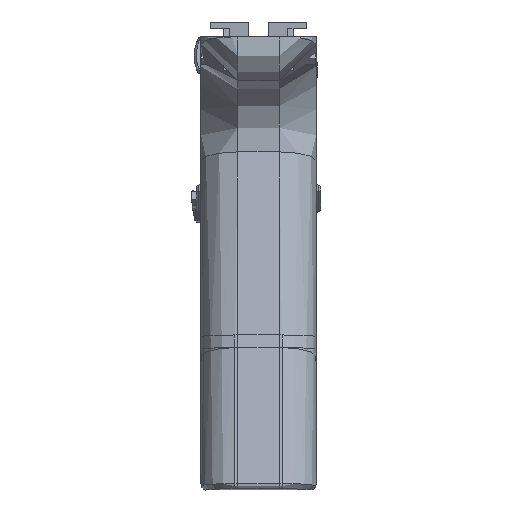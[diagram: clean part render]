
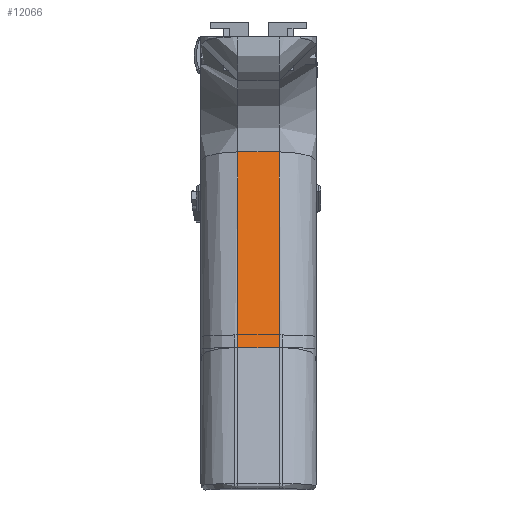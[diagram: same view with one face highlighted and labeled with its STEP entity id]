
A CAD part, front view. The second image highlights one B-rep face of the part: STEP entity #12066.
In plain terms, the highlighted face is planar.
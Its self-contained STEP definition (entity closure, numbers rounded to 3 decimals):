
#883=PLANE('',#13196);
#1446=FACE_OUTER_BOUND('',#2139,.T.);
#2139=EDGE_LOOP('',(#10403,#10404,#10405,#10406));
#3026=LINE('',#21189,#4119);
#3185=LINE('',#22046,#4278);
#3186=LINE('',#22049,#4279);
#3187=LINE('',#22050,#4280);
#4119=VECTOR('',#15585,10.);
#4278=VECTOR('',#15992,10.);
#4279=VECTOR('',#15995,10.);
#4280=VECTOR('',#15996,10.);
#5628=VERTEX_POINT('',#21185);
#5629=VERTEX_POINT('',#21187);
#5770=VERTEX_POINT('',#22024);
#5773=VERTEX_POINT('',#22048);
#7164=EDGE_CURVE('',#5628,#5629,#3026,.T.);
#7393=EDGE_CURVE('',#5628,#5770,#3185,.T.);
#7394=EDGE_CURVE('',#5773,#5629,#3186,.T.);
#7395=EDGE_CURVE('',#5770,#5773,#3187,.T.);
#10403=ORIENTED_EDGE('',*,*,#7394,.F.);
#10404=ORIENTED_EDGE('',*,*,#7395,.F.);
#10405=ORIENTED_EDGE('',*,*,#7393,.F.);
#10406=ORIENTED_EDGE('',*,*,#7164,.T.);
#12066=ADVANCED_FACE('',(#1446),#883,.T.);
#13196=AXIS2_PLACEMENT_3D('',#22047,#15993,#15994);
#15585=DIRECTION('',(0.,-0.249,0.969));
#15992=DIRECTION('',(-1.,0.,0.));
#15993=DIRECTION('center_axis',(0.,-0.969,
-0.249));
#15994=DIRECTION('ref_axis',(0.,-0.249,0.969));
#15995=DIRECTION('',(1.,0.,0.));
#15996=DIRECTION('',(0.,-0.249,0.969));
#21185=CARTESIAN_POINT('',(13.45,-71.634,19.877));
#21187=CARTESIAN_POINT('',(13.45,-83.628,66.536));
#21189=CARTESIAN_POINT('',(13.45,-83.554,66.245));
#22024=CARTESIAN_POINT('',(3.45,-71.634,19.877));
#22046=CARTESIAN_POINT('',(22.175,-71.634,19.877));
#22047=CARTESIAN_POINT('Origin',(22.175,-71.634,19.877));
#22048=CARTESIAN_POINT('',(3.45,-83.628,66.536));
#22049=CARTESIAN_POINT('',(22.175,-83.628,66.536));
#22050=CARTESIAN_POINT('',(3.45,-83.554,66.245));
